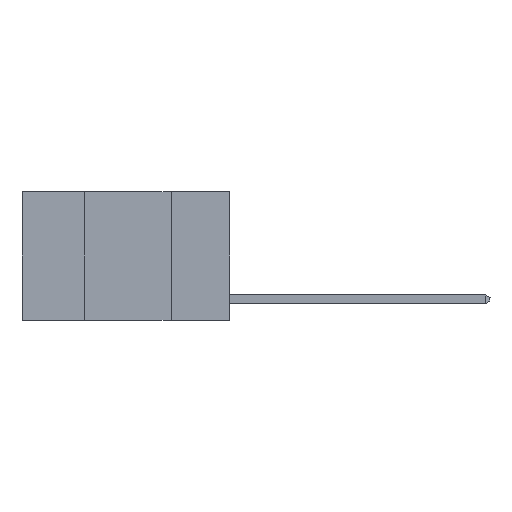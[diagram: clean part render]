
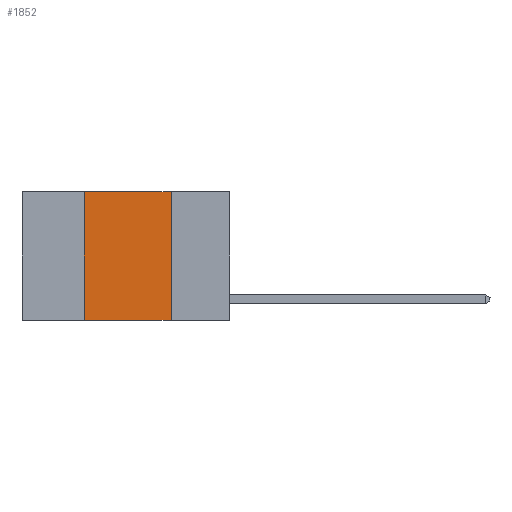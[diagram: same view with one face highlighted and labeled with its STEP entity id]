
A CAD part, left-side view. The second image highlights one B-rep face of the part: STEP entity #1852.
In plain terms, the highlighted planar face has unit normal (-1, 0, 0).
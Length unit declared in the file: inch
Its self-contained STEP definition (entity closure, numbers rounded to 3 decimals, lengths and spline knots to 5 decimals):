
#594 = ORIENTED_EDGE ( 'NONE', *, *, #6473, .F. ) ;
#869 = VECTOR ( 'NONE', #3058, 39.37008 ) ;
#1387 = VECTOR ( 'NONE', #3626, 39.37008 ) ;
#1852 = ADVANCED_FACE ( 'NONE', ( #2726 ), #8107, .F. ) ;
#1961 = CARTESIAN_POINT ( 'NONE',  ( 0., 0.6, 0. ) ) ;
#2090 = LINE ( 'NONE', #11209, #13884 ) ;
#2726 = FACE_OUTER_BOUND ( 'NONE', #10359, .T. ) ;
#2759 = VERTEX_POINT ( 'NONE', #9601 ) ;
#3058 = DIRECTION ( 'NONE',  ( 0., -1., 0. ) ) ;
#3465 = VERTEX_POINT ( 'NONE', #6407 ) ;
#3626 = DIRECTION ( 'NONE',  ( 0., -1., 0. ) ) ;
#4337 = LINE ( 'NONE', #4747, #1387 ) ;
#4747 = CARTESIAN_POINT ( 'NONE',  ( 0., 0.6, -0.37 ) ) ;
#5033 = ORIENTED_EDGE ( 'NONE', *, *, #8914, .F. ) ;
#5053 = CARTESIAN_POINT ( 'NONE',  ( 0., 0.6, 0. ) ) ;
#6407 = CARTESIAN_POINT ( 'NONE',  ( 0., 0.17, -0.37 ) ) ;
#6473 = EDGE_CURVE ( 'NONE', #2759, #3465, #10323, .T. ) ;
#6802 = ORIENTED_EDGE ( 'NONE', *, *, #10063, .F. ) ;
#7104 = VECTOR ( 'NONE', #12552, 39.37008 ) ;
#7176 = CARTESIAN_POINT ( 'NONE',  ( 0., 0.17, 0. ) ) ;
#7391 = AXIS2_PLACEMENT_3D ( 'NONE', #5053, #12756, #10737 ) ;
#7405 = ORIENTED_EDGE ( 'NONE', *, *, #10084, .T. ) ;
#7551 = VERTEX_POINT ( 'NONE', #8516 ) ;
#8107 = PLANE ( 'NONE',  #7391 ) ;
#8516 = CARTESIAN_POINT ( 'NONE',  ( 0., 0.42, 0. ) ) ;
#8914 = EDGE_CURVE ( 'NONE', #7551, #2759, #12127, .T. ) ;
#9601 = CARTESIAN_POINT ( 'NONE',  ( 0., 0.17, 0. ) ) ;
#10040 = DIRECTION ( 'NONE',  ( 0., 0., 1. ) ) ;
#10063 = EDGE_CURVE ( 'NONE', #10834, #7551, #2090, .T. ) ;
#10084 = EDGE_CURVE ( 'NONE', #10834, #3465, #4337, .T. ) ;
#10323 = LINE ( 'NONE', #7176, #7104 ) ;
#10359 = EDGE_LOOP ( 'NONE', ( #594, #5033, #6802, #7405 ) ) ;
#10407 = CARTESIAN_POINT ( 'NONE',  ( 0., 0.42, -0.37 ) ) ;
#10737 = DIRECTION ( 'NONE',  ( 0., 0., -1. ) ) ;
#10834 = VERTEX_POINT ( 'NONE', #10407 ) ;
#11209 = CARTESIAN_POINT ( 'NONE',  ( 0., 0.42, 0. ) ) ;
#12127 = LINE ( 'NONE', #1961, #869 ) ;
#12552 = DIRECTION ( 'NONE',  ( 0., 0., -1. ) ) ;
#12756 = DIRECTION ( 'NONE',  ( 1., 0., 0. ) ) ;
#13884 = VECTOR ( 'NONE', #10040, 39.37008 ) ;
